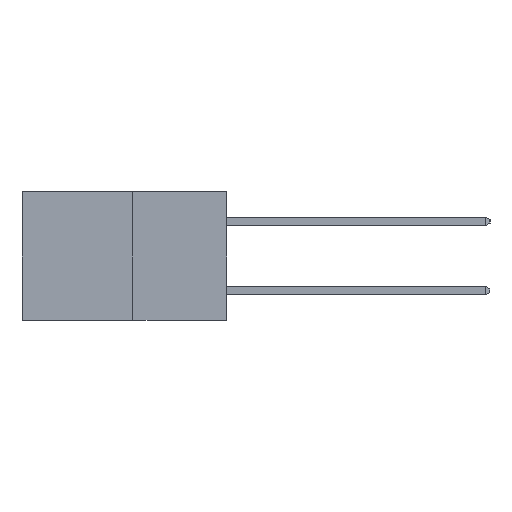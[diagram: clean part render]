
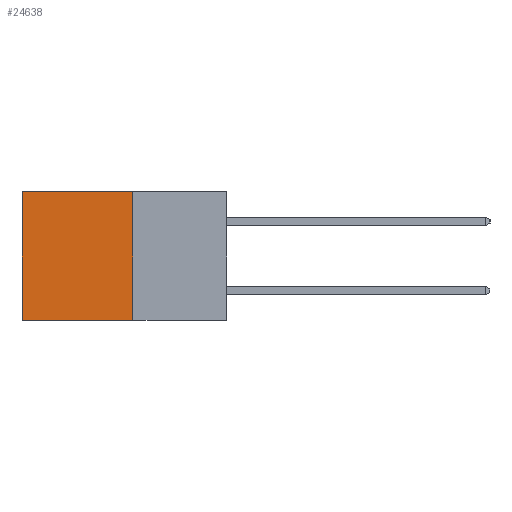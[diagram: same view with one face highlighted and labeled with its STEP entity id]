
A CAD part, left-side view. The second image highlights one B-rep face of the part: STEP entity #24638.
In plain terms, the highlighted planar face has unit normal (-1, 0, 0).
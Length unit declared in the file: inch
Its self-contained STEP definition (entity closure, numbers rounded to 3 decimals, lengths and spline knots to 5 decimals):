
#883 = VECTOR ( 'NONE', #15487, 39.37008 ) ;
#1000 = CARTESIAN_POINT ( 'NONE',  ( 0.277, 0.27, -0.37 ) ) ;
#1307 = ORIENTED_EDGE ( 'NONE', *, *, #19198, .T. ) ;
#2759 = CARTESIAN_POINT ( 'NONE',  ( 0.277, 0.59, -0.37 ) ) ;
#3315 = ORIENTED_EDGE ( 'NONE', *, *, #10932, .F. ) ;
#3979 = VECTOR ( 'NONE', #20984, 39.37008 ) ;
#4626 = VERTEX_POINT ( 'NONE', #7151 ) ;
#7151 = CARTESIAN_POINT ( 'NONE',  ( 0.277, 0.27, 0. ) ) ;
#8746 = EDGE_CURVE ( 'NONE', #26714, #27258, #9859, .T. ) ;
#9859 = LINE ( 'NONE', #1000, #3979 ) ;
#10932 = EDGE_CURVE ( 'NONE', #4626, #26714, #25652, .T. ) ;
#10962 = CARTESIAN_POINT ( 'NONE',  ( 0.277, 0.27, -0.37 ) ) ;
#12082 = VERTEX_POINT ( 'NONE', #14355 ) ;
#14051 = VECTOR ( 'NONE', #22505, 39.37008 ) ;
#14355 = CARTESIAN_POINT ( 'NONE',  ( 0.277, 0.59, 0. ) ) ;
#15049 = CARTESIAN_POINT ( 'NONE',  ( 0.277, 0.27, -0.37 ) ) ;
#15477 = ORIENTED_EDGE ( 'NONE', *, *, #26590, .T. ) ;
#15487 = DIRECTION ( 'NONE',  ( 0., 1., 0. ) ) ;
#15959 = DIRECTION ( 'NONE',  ( 0., 0., -1. ) ) ;
#16007 = VECTOR ( 'NONE', #30208, 39.37008 ) ;
#17172 = AXIS2_PLACEMENT_3D ( 'NONE', #10962, #30772, #15959 ) ;
#19198 = EDGE_CURVE ( 'NONE', #4626, #12082, #20026, .T. ) ;
#20026 = LINE ( 'NONE', #30318, #883 ) ;
#20984 = DIRECTION ( 'NONE',  ( 0., 1., 0. ) ) ;
#22505 = DIRECTION ( 'NONE',  ( 0., 0., -1. ) ) ;
#24638 = ADVANCED_FACE ( 'NONE', ( #29625 ), #25800, .F. ) ;
#25652 = LINE ( 'NONE', #15049, #14051 ) ;
#25657 = CARTESIAN_POINT ( 'NONE',  ( 0.277, 0.27, -0.37 ) ) ;
#25800 = PLANE ( 'NONE',  #17172 ) ;
#26590 = EDGE_CURVE ( 'NONE', #12082, #27258, #29222, .T. ) ;
#26714 = VERTEX_POINT ( 'NONE', #25657 ) ;
#27258 = VERTEX_POINT ( 'NONE', #2759 ) ;
#27733 = CARTESIAN_POINT ( 'NONE',  ( 0.277, 0.59, -0.37 ) ) ;
#28569 = EDGE_LOOP ( 'NONE', ( #15477, #30056, #3315, #1307 ) ) ;
#29222 = LINE ( 'NONE', #27733, #16007 ) ;
#29625 = FACE_OUTER_BOUND ( 'NONE', #28569, .T. ) ;
#30056 = ORIENTED_EDGE ( 'NONE', *, *, #8746, .F. ) ;
#30208 = DIRECTION ( 'NONE',  ( 0., 0., -1. ) ) ;
#30318 = CARTESIAN_POINT ( 'NONE',  ( 0.277, 0.27, 0. ) ) ;
#30772 = DIRECTION ( 'NONE',  ( 1., 0., 0. ) ) ;
